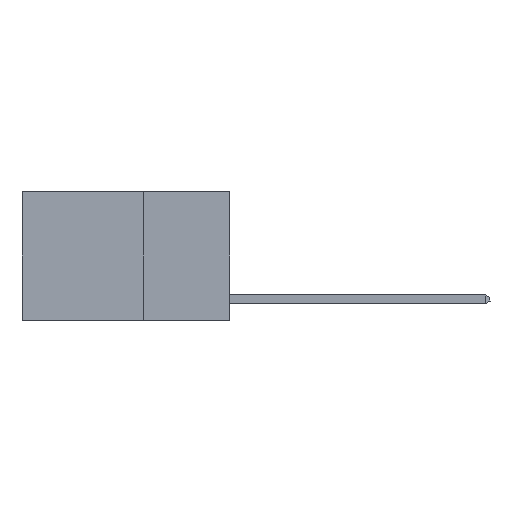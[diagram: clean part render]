
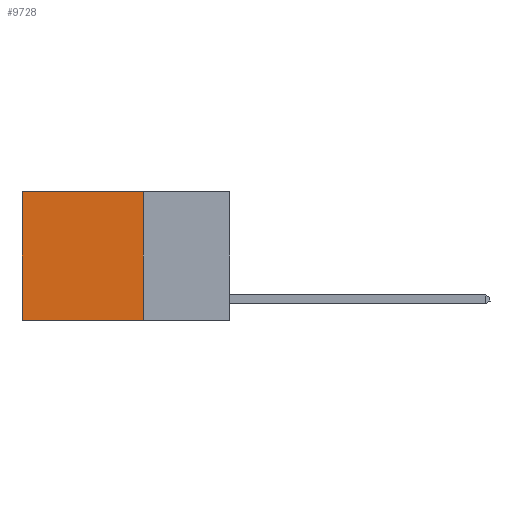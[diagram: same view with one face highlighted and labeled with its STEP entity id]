
A CAD part, left-side view. The second image highlights one B-rep face of the part: STEP entity #9728.
In plain terms, the highlighted planar face has unit normal (-1, 0, 0).
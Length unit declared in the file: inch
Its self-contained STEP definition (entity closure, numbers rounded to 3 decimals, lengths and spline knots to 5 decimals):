
#17 = VECTOR ( 'NONE', #10355, 39.37008 ) ;
#108 = EDGE_CURVE ( 'NONE', #1078, #18396, #1202, .T. ) ;
#977 = CARTESIAN_POINT ( 'NONE',  ( 0.2625, 0.6, -0.37 ) ) ;
#1078 = VERTEX_POINT ( 'NONE', #1103 ) ;
#1103 = CARTESIAN_POINT ( 'NONE',  ( 0.2625, 0.25, 0. ) ) ;
#1202 = LINE ( 'NONE', #21837, #17 ) ;
#2798 = DIRECTION ( 'NONE',  ( 0., 1., 0. ) ) ;
#3635 = EDGE_CURVE ( 'NONE', #16906, #13054, #5951, .T. ) ;
#4250 = CARTESIAN_POINT ( 'NONE',  ( 0.2625, 0.25, -0.37 ) ) ;
#4753 = DIRECTION ( 'NONE',  ( 1., 0., 0. ) ) ;
#5934 = CARTESIAN_POINT ( 'NONE',  ( 0.2625, 0.6, 0. ) ) ;
#5951 = LINE ( 'NONE', #12086, #20106 ) ;
#6716 = ORIENTED_EDGE ( 'NONE', *, *, #7256, .F. ) ;
#7256 = EDGE_CURVE ( 'NONE', #1078, #16906, #12132, .T. ) ;
#7900 = CARTESIAN_POINT ( 'NONE',  ( 0.2625, 0.6, 0. ) ) ;
#7927 = ORIENTED_EDGE ( 'NONE', *, *, #18409, .T. ) ;
#9111 = FACE_OUTER_BOUND ( 'NONE', #14994, .T. ) ;
#9655 = VECTOR ( 'NONE', #13510, 39.37008 ) ;
#9728 = ADVANCED_FACE ( 'NONE', ( #9111 ), #10291, .F. ) ;
#9905 = ORIENTED_EDGE ( 'NONE', *, *, #3635, .F. ) ;
#10267 = DIRECTION ( 'NONE',  ( 0., 0., -1. ) ) ;
#10291 = PLANE ( 'NONE',  #11803 ) ;
#10355 = DIRECTION ( 'NONE',  ( 0., 1., 0. ) ) ;
#11803 = AXIS2_PLACEMENT_3D ( 'NONE', #15883, #4753, #17749 ) ;
#12086 = CARTESIAN_POINT ( 'NONE',  ( 0.2625, 0.25, -0.37 ) ) ;
#12132 = LINE ( 'NONE', #17638, #16450 ) ;
#13054 = VERTEX_POINT ( 'NONE', #977 ) ;
#13510 = DIRECTION ( 'NONE',  ( 0., 0., -1. ) ) ;
#14994 = EDGE_LOOP ( 'NONE', ( #7927, #9905, #6716, #22458 ) ) ;
#15883 = CARTESIAN_POINT ( 'NONE',  ( 0.2625, 0.25, 0. ) ) ;
#16450 = VECTOR ( 'NONE', #10267, 39.37008 ) ;
#16906 = VERTEX_POINT ( 'NONE', #4250 ) ;
#17638 = CARTESIAN_POINT ( 'NONE',  ( 0.2625, 0.25, 0. ) ) ;
#17749 = DIRECTION ( 'NONE',  ( 0., 0., -1. ) ) ;
#18396 = VERTEX_POINT ( 'NONE', #7900 ) ;
#18409 = EDGE_CURVE ( 'NONE', #18396, #13054, #19503, .T. ) ;
#19503 = LINE ( 'NONE', #5934, #9655 ) ;
#20106 = VECTOR ( 'NONE', #2798, 39.37008 ) ;
#21837 = CARTESIAN_POINT ( 'NONE',  ( 0.2625, 0.25, 0. ) ) ;
#22458 = ORIENTED_EDGE ( 'NONE', *, *, #108, .T. ) ;
